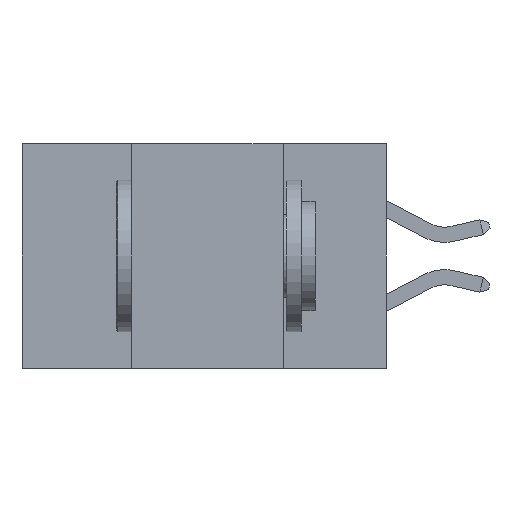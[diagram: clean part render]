
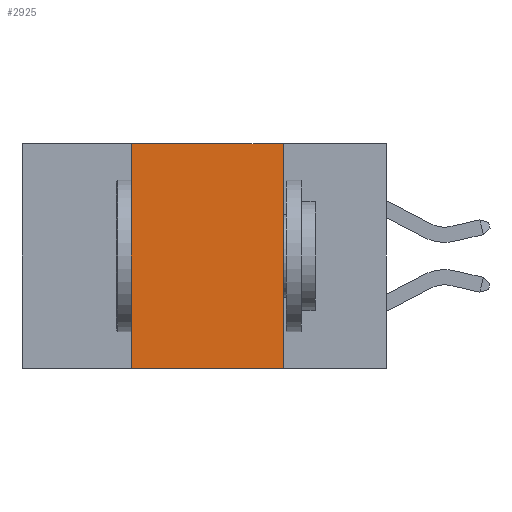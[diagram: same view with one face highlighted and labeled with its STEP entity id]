
A CAD part, left-side view. The second image highlights one B-rep face of the part: STEP entity #2925.
In plain terms, the highlighted planar face has unit normal (-1, 0, 0).
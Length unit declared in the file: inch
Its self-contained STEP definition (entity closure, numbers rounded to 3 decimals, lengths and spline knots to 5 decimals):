
#348 = CARTESIAN_POINT ( 'NONE',  ( 0., 0.42, -0.37 ) ) ;
#461 = ORIENTED_EDGE ( 'NONE', *, *, #6349, .T. ) ;
#720 = CARTESIAN_POINT ( 'NONE',  ( 0., 0.42, 0. ) ) ;
#998 = VERTEX_POINT ( 'NONE', #720 ) ;
#1062 = DIRECTION ( 'NONE',  ( 0., 0., -1. ) ) ;
#1148 = CARTESIAN_POINT ( 'NONE',  ( 0., 0.17, 0. ) ) ;
#1150 = ORIENTED_EDGE ( 'NONE', *, *, #6753, .F. ) ;
#1224 = LINE ( 'NONE', #6433, #2342 ) ;
#1349 = CARTESIAN_POINT ( 'NONE',  ( 0., 0.6, 0. ) ) ;
#1531 = PLANE ( 'NONE',  #3806 ) ;
#2342 = VECTOR ( 'NONE', #2772, 39.37008 ) ;
#2767 = DIRECTION ( 'NONE',  ( 0., -1., 0. ) ) ;
#2772 = DIRECTION ( 'NONE',  ( 0., -1., 0. ) ) ;
#2925 = ADVANCED_FACE ( 'NONE', ( #5893 ), #1531, .F. ) ;
#3330 = DIRECTION ( 'NONE',  ( 0., 0., 1. ) ) ;
#3801 = CARTESIAN_POINT ( 'NONE',  ( 0., 0.42, -0.37 ) ) ;
#3806 = AXIS2_PLACEMENT_3D ( 'NONE', #6555, #5938, #8912 ) ;
#4275 = CARTESIAN_POINT ( 'NONE',  ( 0., 0.17, -0.37 ) ) ;
#4392 = EDGE_CURVE ( 'NONE', #5336, #4829, #7624, .T. ) ;
#4821 = VECTOR ( 'NONE', #2767, 39.37008 ) ;
#4829 = VERTEX_POINT ( 'NONE', #4275 ) ;
#5336 = VERTEX_POINT ( 'NONE', #1148 ) ;
#5521 = LINE ( 'NONE', #348, #6373 ) ;
#5649 = ORIENTED_EDGE ( 'NONE', *, *, #8839, .F. ) ;
#5893 = FACE_OUTER_BOUND ( 'NONE', #8433, .T. ) ;
#5938 = DIRECTION ( 'NONE',  ( 1., 0., 0. ) ) ;
#6349 = EDGE_CURVE ( 'NONE', #7733, #4829, #1224, .T. ) ;
#6373 = VECTOR ( 'NONE', #3330, 39.37008 ) ;
#6433 = CARTESIAN_POINT ( 'NONE',  ( 0., 0.6, -0.37 ) ) ;
#6555 = CARTESIAN_POINT ( 'NONE',  ( 0., 0.6, 0. ) ) ;
#6595 = VECTOR ( 'NONE', #1062, 39.37008 ) ;
#6753 = EDGE_CURVE ( 'NONE', #998, #5336, #9406, .T. ) ;
#7624 = LINE ( 'NONE', #8404, #6595 ) ;
#7733 = VERTEX_POINT ( 'NONE', #3801 ) ;
#8404 = CARTESIAN_POINT ( 'NONE',  ( 0., 0.17, -0.37 ) ) ;
#8433 = EDGE_LOOP ( 'NONE', ( #8857, #1150, #5649, #461 ) ) ;
#8839 = EDGE_CURVE ( 'NONE', #7733, #998, #5521, .T. ) ;
#8857 = ORIENTED_EDGE ( 'NONE', *, *, #4392, .F. ) ;
#8912 = DIRECTION ( 'NONE',  ( 0., 0., -1. ) ) ;
#9406 = LINE ( 'NONE', #1349, #4821 ) ;
